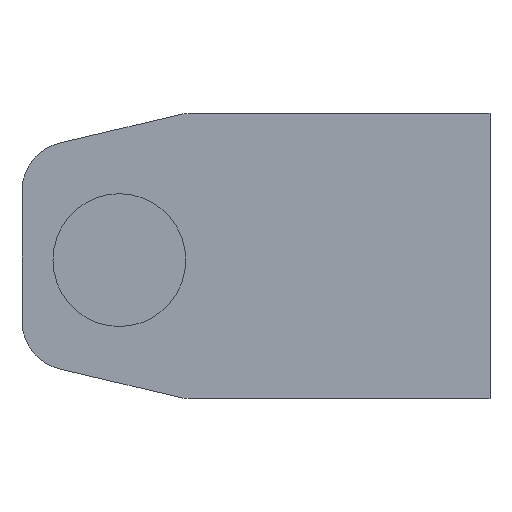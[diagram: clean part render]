
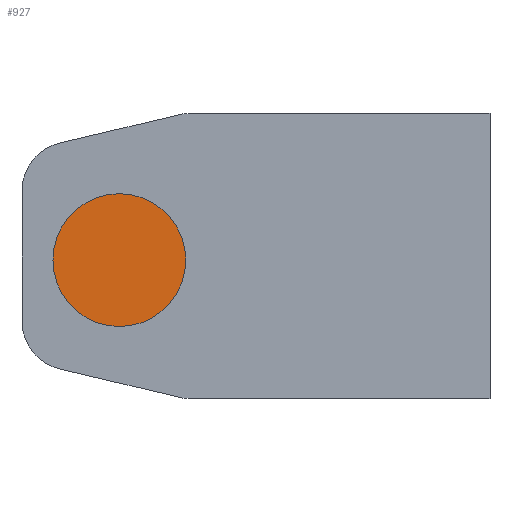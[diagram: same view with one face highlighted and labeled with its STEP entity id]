
A CAD part, front view. The second image highlights one B-rep face of the part: STEP entity #927.
In plain terms, the highlighted planar face has unit normal (0, -1, 0).
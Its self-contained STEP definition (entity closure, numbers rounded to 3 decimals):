
#426 = CYLINDRICAL_SURFACE('',#427,4.3);
#427 = AXIS2_PLACEMENT_3D('',#428,#429,#430);
#428 = CARTESIAN_POINT('',(10.,0.,-14.5));
#429 = DIRECTION('',(0.,1.,0.));
#430 = DIRECTION('',(0.,0.,1.));
#878 = VERTEX_POINT('',#879);
#879 = CARTESIAN_POINT('',(10.,0.,-10.2));
#900 = EDGE_CURVE('',#878,#878,#901,.T.);
#901 = SURFACE_CURVE('',#902,(#907,#914),.PCURVE_S1.);
#902 = CIRCLE('',#903,4.3);
#903 = AXIS2_PLACEMENT_3D('',#904,#905,#906);
#904 = CARTESIAN_POINT('',(10.,0.,-14.5));
#905 = DIRECTION('',(0.,1.,0.));
#906 = DIRECTION('',(0.,0.,1.));
#907 = PCURVE('',#426,#908);
#908 = DEFINITIONAL_REPRESENTATION('',(#909),#913);
#909 = LINE('',#910,#911);
#910 = CARTESIAN_POINT('',(0.,0.));
#911 = VECTOR('',#912,1.);
#912 = DIRECTION('',(1.,0.));
#913 = ( GEOMETRIC_REPRESENTATION_CONTEXT(2) 
PARAMETRIC_REPRESENTATION_CONTEXT() REPRESENTATION_CONTEXT('2D SPACE',''
  ) );
#914 = PCURVE('',#915,#920);
#915 = PLANE('',#916);
#916 = AXIS2_PLACEMENT_3D('',#917,#918,#919);
#917 = CARTESIAN_POINT('',(10.,0.,-14.5));
#918 = DIRECTION('',(0.,1.,0.));
#919 = DIRECTION('',(0.,0.,1.));
#920 = DEFINITIONAL_REPRESENTATION('',(#921),#925);
#921 = CIRCLE('',#922,4.3);
#922 = AXIS2_PLACEMENT_2D('',#923,#924);
#923 = CARTESIAN_POINT('',(0.,0.));
#924 = DIRECTION('',(1.,0.));
#925 = ( GEOMETRIC_REPRESENTATION_CONTEXT(2) 
PARAMETRIC_REPRESENTATION_CONTEXT() REPRESENTATION_CONTEXT('2D SPACE',''
  ) );
#927 = ADVANCED_FACE('',(#928),#915,.F.);
#928 = FACE_BOUND('',#929,.T.);
#929 = EDGE_LOOP('',(#930));
#930 = ORIENTED_EDGE('',*,*,#900,.F.);
